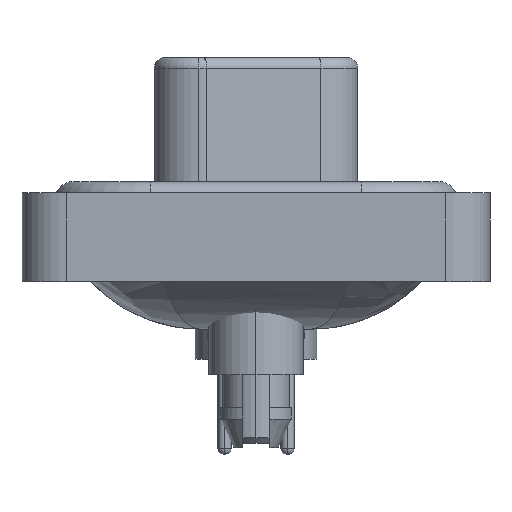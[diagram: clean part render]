
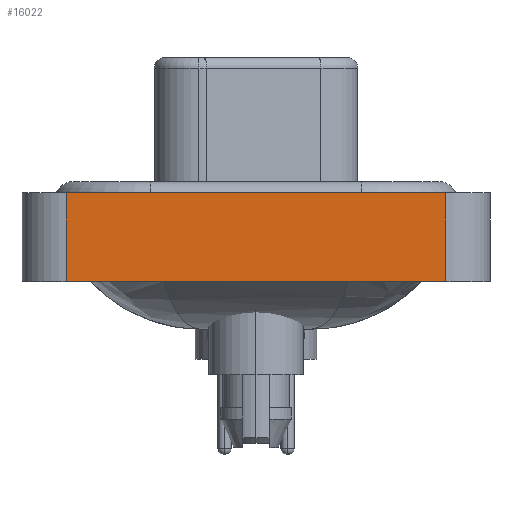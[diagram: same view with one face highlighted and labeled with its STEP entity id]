
A CAD part, left-side view. The second image highlights one B-rep face of the part: STEP entity #16022.
In plain terms, the highlighted planar face has unit normal (-1, 0, 0).
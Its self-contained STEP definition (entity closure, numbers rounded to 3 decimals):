
#566 = ORIENTED_EDGE ( 'NONE', *, *, #23054, .T. ) ;
#1575 = CARTESIAN_POINT ( 'NONE',  ( -7.35, -8.55, -3.6 ) ) ;
#2918 = VECTOR ( 'NONE', #12493, 1000. ) ;
#3298 = EDGE_CURVE ( 'NONE', #10897, #15702, #14243, .T. ) ;
#3356 = CARTESIAN_POINT ( 'NONE',  ( -7.35, 8.55, -3.6 ) ) ;
#3451 = AXIS2_PLACEMENT_3D ( 'NONE', #19206, #11867, #23262 ) ;
#3768 = VERTEX_POINT ( 'NONE', #19540 ) ;
#4137 = FACE_OUTER_BOUND ( 'NONE', #5052, .T. ) ;
#4630 = CARTESIAN_POINT ( 'NONE',  ( -7.35, -8.55, 0.4 ) ) ;
#5052 = EDGE_LOOP ( 'NONE', ( #13818, #9699, #5456, #566 ) ) ;
#5193 = VERTEX_POINT ( 'NONE', #5661 ) ;
#5456 = ORIENTED_EDGE ( 'NONE', *, *, #8108, .F. ) ;
#5661 = CARTESIAN_POINT ( 'NONE',  ( -7.35, -8.55, -3.6 ) ) ;
#6828 = LINE ( 'NONE', #24412, #16372 ) ;
#7062 = LINE ( 'NONE', #3356, #12564 ) ;
#7079 = DIRECTION ( 'NONE',  ( 0., 0., 1. ) ) ;
#8108 = EDGE_CURVE ( 'NONE', #3768, #10897, #7062, .T. ) ;
#8364 = CARTESIAN_POINT ( 'NONE',  ( -7.35, -8.55, 0.4 ) ) ;
#9699 = ORIENTED_EDGE ( 'NONE', *, *, #3298, .F. ) ;
#10897 = VERTEX_POINT ( 'NONE', #12796 ) ;
#11867 = DIRECTION ( 'NONE',  ( -1., 0., 0. ) ) ;
#12493 = DIRECTION ( 'NONE',  ( 0., -1., 0. ) ) ;
#12564 = VECTOR ( 'NONE', #14770, 1000. ) ;
#12796 = CARTESIAN_POINT ( 'NONE',  ( -7.35, 8.55, 0.4 ) ) ;
#13818 = ORIENTED_EDGE ( 'NONE', *, *, #14860, .T. ) ;
#14243 = LINE ( 'NONE', #4630, #2918 ) ;
#14770 = DIRECTION ( 'NONE',  ( 0., 0., 1. ) ) ;
#14860 = EDGE_CURVE ( 'NONE', #5193, #15702, #6828, .T. ) ;
#15702 = VERTEX_POINT ( 'NONE', #8364 ) ;
#16022 = ADVANCED_FACE ( 'NONE', ( #4137 ), #23004, .T. ) ;
#16372 = VECTOR ( 'NONE', #7079, 1000. ) ;
#17302 = LINE ( 'NONE', #1575, #17733 ) ;
#17733 = VECTOR ( 'NONE', #25001, 1000. ) ;
#19206 = CARTESIAN_POINT ( 'NONE',  ( -7.35, -8.55, -3.6 ) ) ;
#19540 = CARTESIAN_POINT ( 'NONE',  ( -7.35, 8.55, -3.6 ) ) ;
#23004 = PLANE ( 'NONE',  #3451 ) ;
#23054 = EDGE_CURVE ( 'NONE', #3768, #5193, #17302, .T. ) ;
#23262 = DIRECTION ( 'NONE',  ( 0., 0., 1. ) ) ;
#24412 = CARTESIAN_POINT ( 'NONE',  ( -7.35, -8.55, -3.6 ) ) ;
#25001 = DIRECTION ( 'NONE',  ( 0., -1., 0. ) ) ;
